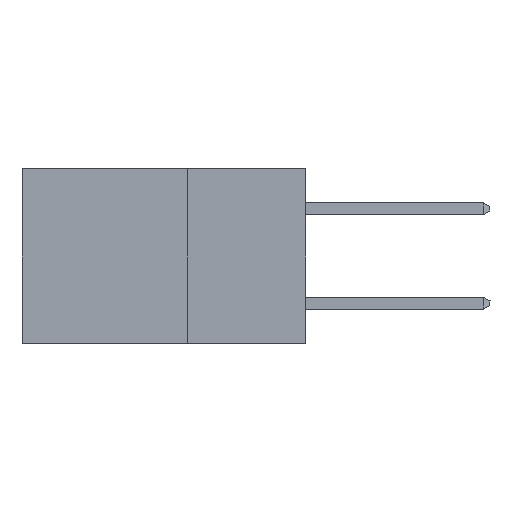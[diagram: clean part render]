
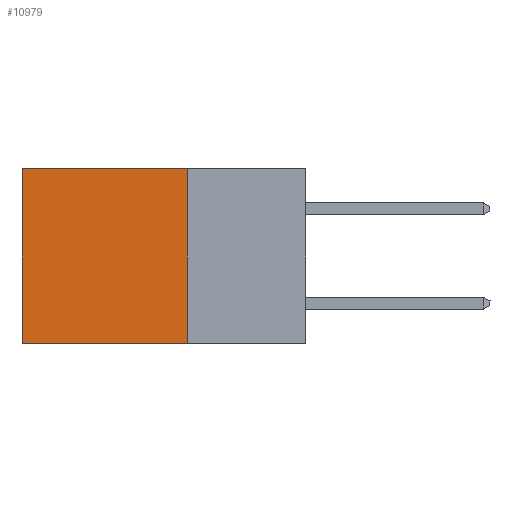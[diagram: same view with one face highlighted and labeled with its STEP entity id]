
A CAD part, left-side view. The second image highlights one B-rep face of the part: STEP entity #10979.
In plain terms, the highlighted planar face has unit normal (-1, 0, 0).
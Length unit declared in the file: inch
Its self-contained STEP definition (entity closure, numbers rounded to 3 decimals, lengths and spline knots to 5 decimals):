
#157 = CARTESIAN_POINT ( 'NONE',  ( 0.2615, 0.25, -0.37 ) ) ;
#749 = ORIENTED_EDGE ( 'NONE', *, *, #5042, .T. ) ;
#875 = CARTESIAN_POINT ( 'NONE',  ( 0.2615, 0.25, 0. ) ) ;
#1308 = CARTESIAN_POINT ( 'NONE',  ( 0.2615, 0.6, 0. ) ) ;
#1351 = PLANE ( 'NONE',  #22604 ) ;
#1676 = ORIENTED_EDGE ( 'NONE', *, *, #22308, .T. ) ;
#4630 = CARTESIAN_POINT ( 'NONE',  ( 0.2615, 0.25, -0.37 ) ) ;
#4934 = LINE ( 'NONE', #14796, #9784 ) ;
#5042 = EDGE_CURVE ( 'NONE', #10779, #23204, #4934, .T. ) ;
#5658 = ORIENTED_EDGE ( 'NONE', *, *, #23091, .F. ) ;
#6157 = LINE ( 'NONE', #4630, #15278 ) ;
#6477 = DIRECTION ( 'NONE',  ( 0., 1., 0. ) ) ;
#6785 = EDGE_LOOP ( 'NONE', ( #1676, #5658, #20100, #749 ) ) ;
#6832 = DIRECTION ( 'NONE',  ( 1., 0., 0. ) ) ;
#8753 = LINE ( 'NONE', #10620, #17861 ) ;
#9784 = VECTOR ( 'NONE', #22008, 39.37008 ) ;
#10620 = CARTESIAN_POINT ( 'NONE',  ( 0.2615, 0.25, -0.37 ) ) ;
#10779 = VERTEX_POINT ( 'NONE', #875 ) ;
#10979 = ADVANCED_FACE ( 'NONE', ( #12659 ), #1351, .F. ) ;
#11687 = CARTESIAN_POINT ( 'NONE',  ( 0.2615, 0.6, -0.37 ) ) ;
#12450 = DIRECTION ( 'NONE',  ( 0., 0., -1. ) ) ;
#12487 = VECTOR ( 'NONE', #15328, 39.37008 ) ;
#12659 = FACE_OUTER_BOUND ( 'NONE', #6785, .T. ) ;
#13780 = CARTESIAN_POINT ( 'NONE',  ( 0.2615, 0.6, -0.37 ) ) ;
#13887 = EDGE_CURVE ( 'NONE', #10779, #19679, #8753, .T. ) ;
#14796 = CARTESIAN_POINT ( 'NONE',  ( 0.2615, 0.25, 0. ) ) ;
#15278 = VECTOR ( 'NONE', #6477, 39.37008 ) ;
#15328 = DIRECTION ( 'NONE',  ( 0., 0., -1. ) ) ;
#17743 = CARTESIAN_POINT ( 'NONE',  ( 0.2615, 0.25, -0.37 ) ) ;
#17861 = VECTOR ( 'NONE', #12450, 39.37008 ) ;
#19541 = DIRECTION ( 'NONE',  ( 0., 0., -1. ) ) ;
#19679 = VERTEX_POINT ( 'NONE', #157 ) ;
#20100 = ORIENTED_EDGE ( 'NONE', *, *, #13887, .F. ) ;
#22008 = DIRECTION ( 'NONE',  ( 0., 1., 0. ) ) ;
#22046 = LINE ( 'NONE', #11687, #12487 ) ;
#22308 = EDGE_CURVE ( 'NONE', #23204, #22384, #22046, .T. ) ;
#22384 = VERTEX_POINT ( 'NONE', #13780 ) ;
#22604 = AXIS2_PLACEMENT_3D ( 'NONE', #17743, #6832, #19541 ) ;
#23091 = EDGE_CURVE ( 'NONE', #19679, #22384, #6157, .T. ) ;
#23204 = VERTEX_POINT ( 'NONE', #1308 ) ;
